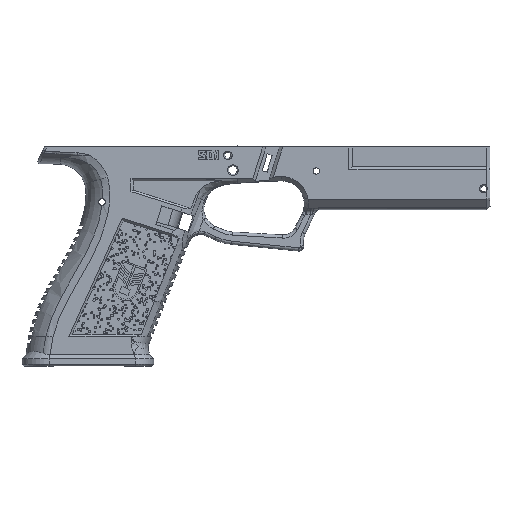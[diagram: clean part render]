
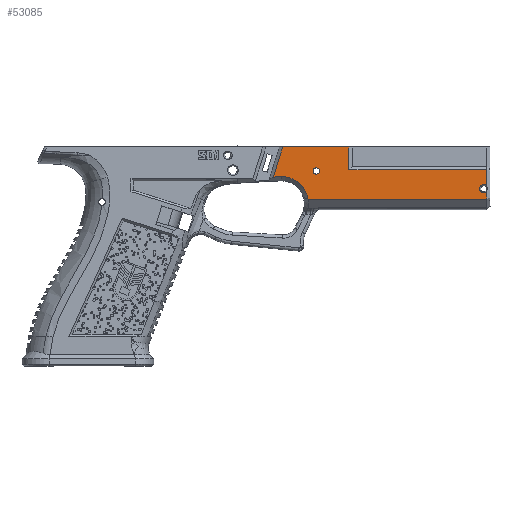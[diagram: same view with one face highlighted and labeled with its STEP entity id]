
A CAD part, front view. The second image highlights one B-rep face of the part: STEP entity #53085.
In plain terms, the highlighted planar face has unit normal (0, -1, 0).
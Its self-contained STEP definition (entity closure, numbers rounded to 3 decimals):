
#5897=FACE_BOUND('',#9899,.T.);
#6455=CIRCLE('',#56363,13.);
#6456=CIRCLE('',#56364,2.);
#6457=CIRCLE('',#56365,1.5);
#6649=FACE_OUTER_BOUND('',#9898,.T.);
#9898=EDGE_LOOP('',(#35612,#35613,#35614,#35615,#35616,#35617,#35618,#35619,
#35620,#35621));
#9899=EDGE_LOOP('',(#35622));
#14837=LINE('',#68584,#18141);
#14869=LINE('',#68664,#18173);
#14870=LINE('',#68666,#18174);
#14871=LINE('',#68670,#18175);
#14872=LINE('',#68672,#18176);
#14873=LINE('',#68676,#18177);
#14874=LINE('',#68678,#18178);
#14875=LINE('',#68679,#18179);
#18141=VECTOR('',#57684,10.);
#18173=VECTOR('',#57730,10.);
#18174=VECTOR('',#57731,10.);
#18175=VECTOR('',#57734,10.);
#18176=VECTOR('',#57735,10.);
#18177=VECTOR('',#57738,10.);
#18178=VECTOR('',#57739,10.);
#18179=VECTOR('',#57740,10.);
#21524=VERTEX_POINT('',#68581);
#21525=VERTEX_POINT('',#68583);
#21554=VERTEX_POINT('',#68663);
#21555=VERTEX_POINT('',#68665);
#21556=VERTEX_POINT('',#68667);
#21557=VERTEX_POINT('',#68669);
#21558=VERTEX_POINT('',#68671);
#21559=VERTEX_POINT('',#68673);
#21560=VERTEX_POINT('',#68675);
#21561=VERTEX_POINT('',#68677);
#21562=VERTEX_POINT('',#68680);
#27095=EDGE_CURVE('',#21525,#21524,#14837,.T.);
#27131=EDGE_CURVE('',#21554,#21524,#14869,.T.);
#27132=EDGE_CURVE('',#21555,#21554,#14870,.T.);
#27133=EDGE_CURVE('',#21556,#21555,#6455,.T.);
#27134=EDGE_CURVE('',#21557,#21556,#14871,.T.);
#27135=EDGE_CURVE('',#21558,#21557,#14872,.T.);
#27136=EDGE_CURVE('',#21559,#21558,#6456,.T.);
#27137=EDGE_CURVE('',#21560,#21559,#14873,.T.);
#27138=EDGE_CURVE('',#21560,#21561,#14874,.T.);
#27139=EDGE_CURVE('',#21525,#21561,#14875,.T.);
#27140=EDGE_CURVE('',#21562,#21562,#6457,.T.);
#35612=ORIENTED_EDGE('',*,*,#27095,.T.);
#35613=ORIENTED_EDGE('',*,*,#27131,.F.);
#35614=ORIENTED_EDGE('',*,*,#27132,.F.);
#35615=ORIENTED_EDGE('',*,*,#27133,.F.);
#35616=ORIENTED_EDGE('',*,*,#27134,.F.);
#35617=ORIENTED_EDGE('',*,*,#27135,.F.);
#35618=ORIENTED_EDGE('',*,*,#27136,.F.);
#35619=ORIENTED_EDGE('',*,*,#27137,.F.);
#35620=ORIENTED_EDGE('',*,*,#27138,.T.);
#35621=ORIENTED_EDGE('',*,*,#27139,.F.);
#35622=ORIENTED_EDGE('',*,*,#27140,.T.);
#52141=PLANE('',#56362);
#53085=ADVANCED_FACE('',(#6649,#5897),#52141,.F.);
#56362=AXIS2_PLACEMENT_3D('',#68662,#57728,#57729);
#56363=AXIS2_PLACEMENT_3D('',#68668,#57732,#57733);
#56364=AXIS2_PLACEMENT_3D('',#68674,#57736,#57737);
#56365=AXIS2_PLACEMENT_3D('',#68681,#57741,#57742);
#57684=DIRECTION('',(-1.,0.,0.));
#57728=DIRECTION('center_axis',(0.,1.,0.));
#57729=DIRECTION('ref_axis',(0.,0.,
1.));
#57730=DIRECTION('',(0.301,0.,0.954));
#57731=DIRECTION('',(-0.999,0.,-0.055));
#57732=DIRECTION('center_axis',(0.,-1.,0.));
#57733=DIRECTION('ref_axis',(0.892,0.,-0.452));
#57734=DIRECTION('',(-1.,0.,0.));
#57735=DIRECTION('',(0.,0.,-1.));
#57736=DIRECTION('center_axis',(0.,-1.,0.));
#57737=DIRECTION('ref_axis',(-1.,0.,0.));
#57738=DIRECTION('',(0.,0.,-1.));
#57739=DIRECTION('',(-1.,0.,0.));
#57740=DIRECTION('',(0.,0.,-1.));
#57741=DIRECTION('center_axis',(0.,1.,0.));
#57742=DIRECTION('ref_axis',(1.,0.,0.));
#68581=CARTESIAN_POINT('',(80.915,-215.077,16.843));
#68583=CARTESIAN_POINT('',(112.635,-215.077,16.843));
#68584=CARTESIAN_POINT('',(37.842,-215.077,16.843));
#68662=CARTESIAN_POINT('Origin',(103.31,-215.077,16.95));
#68663=CARTESIAN_POINT('',(76.374,-215.077,2.443));
#68664=CARTESIAN_POINT('',(80.837,-215.077,16.595));
#68665=CARTESIAN_POINT('',(80.217,-215.077,2.654));
#68666=CARTESIAN_POINT('',(81.633,-215.077,2.731));
#68667=CARTESIAN_POINT('',(93.078,-215.077,-8.096));
#68668=CARTESIAN_POINT('Origin',(80.274,-215.077,-10.346));
#68669=CARTESIAN_POINT('',(178.635,-215.077,-8.096));
#68670=CARTESIAN_POINT('',(89.618,-215.077,-8.096));
#68671=CARTESIAN_POINT('',(178.635,-215.077,-4.419));
#68672=CARTESIAN_POINT('',(178.635,-215.077,-9.397));
#68673=CARTESIAN_POINT('',(178.635,-215.077,-1.773));
#68674=CARTESIAN_POINT('Origin',(177.135,-215.077,-3.096));
#68675=CARTESIAN_POINT('',(178.635,-215.077,5.957));
#68676=CARTESIAN_POINT('',(178.635,-215.077,-9.397));
#68677=CARTESIAN_POINT('',(112.635,-215.077,5.957));
#68678=CARTESIAN_POINT('',(105.549,-215.077,5.957));
#68679=CARTESIAN_POINT('',(112.635,-215.077,17.203));
#68680=CARTESIAN_POINT('',(95.518,-215.077,5.35));
#68681=CARTESIAN_POINT('Origin',(97.018,-215.077,5.35));
